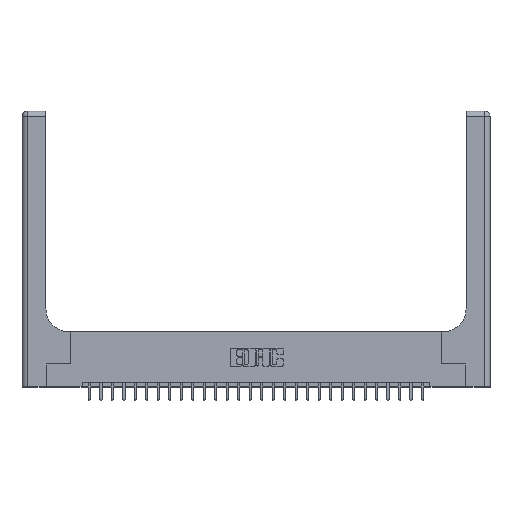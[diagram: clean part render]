
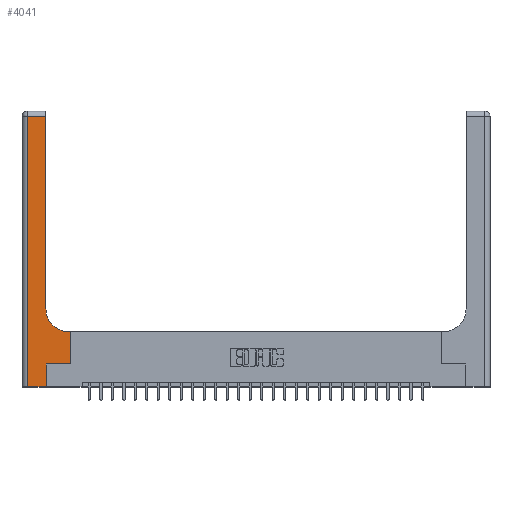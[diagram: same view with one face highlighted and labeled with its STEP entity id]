
A CAD part, top view. The second image highlights one B-rep face of the part: STEP entity #4041.
In plain terms, the highlighted planar face has unit normal (0, 0, 1).
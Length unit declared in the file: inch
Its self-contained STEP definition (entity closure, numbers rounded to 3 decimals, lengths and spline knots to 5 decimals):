
#300 = PLANE ( 'NONE',  #17597 ) ;
#389 = CARTESIAN_POINT ( 'NONE',  ( 0., 3., 0.37 ) ) ;
#1605 = DIRECTION ( 'NONE',  ( 1., 0., 0. ) ) ;
#1858 = DIRECTION ( 'NONE',  ( 1., 0., 0. ) ) ;
#2239 = VECTOR ( 'NONE', #26213, 39.37008 ) ;
#2610 = ORIENTED_EDGE ( 'NONE', *, *, #25480, .T. ) ;
#2882 = LINE ( 'NONE', #8776, #13744 ) ;
#3023 = CARTESIAN_POINT ( 'NONE',  ( 0.265, 0.25, 0.37 ) ) ;
#4041 = ADVANCED_FACE ( 'NONE', ( #8904 ), #300, .F. ) ;
#4043 = VERTEX_POINT ( 'NONE', #14734 ) ;
#4524 = DIRECTION ( 'NONE',  ( -1., 0., 0. ) ) ;
#4675 = DIRECTION ( 'NONE',  ( 0., 1., 0. ) ) ;
#4792 = ORIENTED_EDGE ( 'NONE', *, *, #18977, .T. ) ;
#4920 = EDGE_CURVE ( 'NONE', #18603, #21692, #26107, .T. ) ;
#5056 = DIRECTION ( 'NONE',  ( -1., 0., 0. ) ) ;
#5541 = ORIENTED_EDGE ( 'NONE', *, *, #11328, .T. ) ;
#5790 = LINE ( 'NONE', #12116, #2239 ) ;
#6718 = DIRECTION ( 'NONE',  ( 1., 0., 0. ) ) ;
#7980 = CARTESIAN_POINT ( 'NONE',  ( 0.26, 0.6, 0.37 ) ) ;
#8314 = CARTESIAN_POINT ( 'NONE',  ( 0.528, 0.25, 0.37 ) ) ;
#8574 = DIRECTION ( 'NONE',  ( 0., 1., 0. ) ) ;
#8776 = CARTESIAN_POINT ( 'NONE',  ( 0.265, 0., 0.37 ) ) ;
#8904 = FACE_OUTER_BOUND ( 'NONE', #18247, .T. ) ;
#9426 = CARTESIAN_POINT ( 'NONE',  ( 0.26, 2.94, 0.37 ) ) ;
#9750 = LINE ( 'NONE', #18994, #14198 ) ;
#10298 = VERTEX_POINT ( 'NONE', #20521 ) ;
#11328 = EDGE_CURVE ( 'NONE', #25154, #10298, #5790, .T. ) ;
#11375 = DIRECTION ( 'NONE',  ( 0., 1., 0. ) ) ;
#11479 = CARTESIAN_POINT ( 'NONE',  ( 0.51, 0.6, 0.37 ) ) ;
#11765 = LINE ( 'NONE', #7980, #13332 ) ;
#12116 = CARTESIAN_POINT ( 'NONE',  ( 0.06, 3., 0.37 ) ) ;
#12839 = VECTOR ( 'NONE', #8574, 39.37008 ) ;
#12973 = LINE ( 'NONE', #24754, #13618 ) ;
#13087 = ORIENTED_EDGE ( 'NONE', *, *, #18260, .T. ) ;
#13184 = ORIENTED_EDGE ( 'NONE', *, *, #19139, .T. ) ;
#13332 = VECTOR ( 'NONE', #26353, 39.37008 ) ;
#13618 = VECTOR ( 'NONE', #4524, 39.37008 ) ;
#13744 = VECTOR ( 'NONE', #11375, 39.37008 ) ;
#14198 = VECTOR ( 'NONE', #4675, 39.37008 ) ;
#14734 = CARTESIAN_POINT ( 'NONE',  ( 0.265, 0., 0.37 ) ) ;
#14735 = LINE ( 'NONE', #8314, #12839 ) ;
#15466 = EDGE_CURVE ( 'NONE', #26172, #22255, #16385, .T. ) ;
#16024 = DIRECTION ( 'NONE',  ( 0., 0., -1. ) ) ;
#16033 = VERTEX_POINT ( 'NONE', #18879 ) ;
#16385 = LINE ( 'NONE', #18908, #23752 ) ;
#17079 = CARTESIAN_POINT ( 'NONE',  ( 0.06, 2.94, 0.37 ) ) ;
#17334 = ORIENTED_EDGE ( 'NONE', *, *, #23853, .T. ) ;
#17597 = AXIS2_PLACEMENT_3D ( 'NONE', #389, #22862, #5056 ) ;
#17747 = CARTESIAN_POINT ( 'NONE',  ( 0., 0., 0.37 ) ) ;
#18147 = ORIENTED_EDGE ( 'NONE', *, *, #4920, .T. ) ;
#18247 = EDGE_LOOP ( 'NONE', ( #4792, #13087, #5541, #13184, #17334, #25644, #22075, #2610, #18147 ) ) ;
#18260 = EDGE_CURVE ( 'NONE', #20844, #25154, #12973, .T. ) ;
#18603 = VERTEX_POINT ( 'NONE', #11479 ) ;
#18875 = CARTESIAN_POINT ( 'NONE',  ( 0.528, 0.25, 0.37 ) ) ;
#18879 = CARTESIAN_POINT ( 'NONE',  ( 0.528, 0.6, 0.37 ) ) ;
#18908 = CARTESIAN_POINT ( 'NONE',  ( 0.265, 0.25, 0.37 ) ) ;
#18973 = VECTOR ( 'NONE', #1605, 39.37008 ) ;
#18977 = EDGE_CURVE ( 'NONE', #21692, #20844, #9750, .T. ) ;
#18990 = CARTESIAN_POINT ( 'NONE',  ( 0.26, 0.85, 0.37 ) ) ;
#18994 = CARTESIAN_POINT ( 'NONE',  ( 0.26, 3., 0.37 ) ) ;
#19139 = EDGE_CURVE ( 'NONE', #10298, #4043, #20902, .T. ) ;
#20042 = CARTESIAN_POINT ( 'NONE',  ( 0.51, 0.85, 0.37 ) ) ;
#20521 = CARTESIAN_POINT ( 'NONE',  ( 0.06, 0., 0.37 ) ) ;
#20844 = VERTEX_POINT ( 'NONE', #9426 ) ;
#20902 = LINE ( 'NONE', #17747, #18973 ) ;
#21499 = EDGE_CURVE ( 'NONE', #22255, #16033, #14735, .T. ) ;
#21692 = VERTEX_POINT ( 'NONE', #18990 ) ;
#22075 = ORIENTED_EDGE ( 'NONE', *, *, #21499, .T. ) ;
#22255 = VERTEX_POINT ( 'NONE', #18875 ) ;
#22862 = DIRECTION ( 'NONE',  ( 0., 0., -1. ) ) ;
#23752 = VECTOR ( 'NONE', #6718, 39.37008 ) ;
#23853 = EDGE_CURVE ( 'NONE', #4043, #26172, #2882, .T. ) ;
#24754 = CARTESIAN_POINT ( 'NONE',  ( 0., 2.94, 0.37 ) ) ;
#24778 = AXIS2_PLACEMENT_3D ( 'NONE', #20042, #16024, #1858 ) ;
#25154 = VERTEX_POINT ( 'NONE', #17079 ) ;
#25480 = EDGE_CURVE ( 'NONE', #16033, #18603, #11765, .T. ) ;
#25644 = ORIENTED_EDGE ( 'NONE', *, *, #15466, .T. ) ;
#26107 = CIRCLE ( 'NONE', #24778, 0.25 ) ;
#26172 = VERTEX_POINT ( 'NONE', #3023 ) ;
#26213 = DIRECTION ( 'NONE',  ( 0., -1., 0. ) ) ;
#26353 = DIRECTION ( 'NONE',  ( -1., 0., 0. ) ) ;
